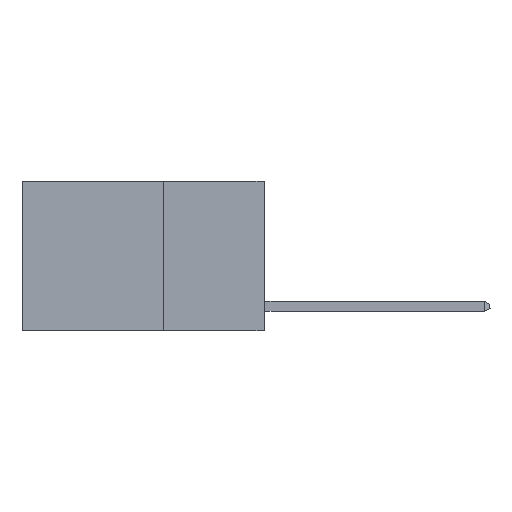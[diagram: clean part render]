
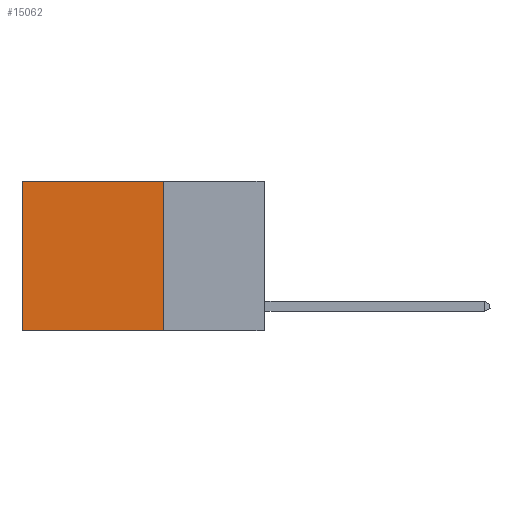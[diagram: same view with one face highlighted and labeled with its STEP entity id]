
A CAD part, left-side view. The second image highlights one B-rep face of the part: STEP entity #15062.
In plain terms, the highlighted planar face has unit normal (-1, 0, 0).
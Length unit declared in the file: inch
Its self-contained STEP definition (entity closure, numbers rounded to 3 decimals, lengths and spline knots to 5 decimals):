
#704 = CARTESIAN_POINT ( 'NONE',  ( 0.2625, 0.25, 0. ) ) ;
#871 = VECTOR ( 'NONE', #14915, 39.37008 ) ;
#1615 = ORIENTED_EDGE ( 'NONE', *, *, #5030, .F. ) ;
#2036 = CARTESIAN_POINT ( 'NONE',  ( 0.2625, 0.6, 0. ) ) ;
#3645 = VERTEX_POINT ( 'NONE', #19910 ) ;
#3768 = CARTESIAN_POINT ( 'NONE',  ( 0.2625, 0.25, 0. ) ) ;
#3844 = FACE_OUTER_BOUND ( 'NONE', #17387, .T. ) ;
#3846 = EDGE_CURVE ( 'NONE', #17988, #3645, #8798, .T. ) ;
#3856 = VERTEX_POINT ( 'NONE', #16458 ) ;
#4804 = LINE ( 'NONE', #2036, #16045 ) ;
#4992 = ORIENTED_EDGE ( 'NONE', *, *, #3846, .F. ) ;
#5030 = EDGE_CURVE ( 'NONE', #3645, #3856, #11576, .T. ) ;
#5071 = DIRECTION ( 'NONE',  ( 1., 0., 0. ) ) ;
#5619 = CARTESIAN_POINT ( 'NONE',  ( 0.2625, 0.25, 0. ) ) ;
#5846 = VECTOR ( 'NONE', #10046, 39.37008 ) ;
#6249 = CARTESIAN_POINT ( 'NONE',  ( 0.2625, 0.6, 0. ) ) ;
#6256 = VECTOR ( 'NONE', #14660, 39.37008 ) ;
#6425 = VERTEX_POINT ( 'NONE', #6249 ) ;
#8798 = LINE ( 'NONE', #5619, #5846 ) ;
#9884 = CARTESIAN_POINT ( 'NONE',  ( 0.2625, 0.25, 0. ) ) ;
#10046 = DIRECTION ( 'NONE',  ( 0., 0., -1. ) ) ;
#10089 = DIRECTION ( 'NONE',  ( 0., 0., -1. ) ) ;
#11225 = EDGE_CURVE ( 'NONE', #6425, #3856, #4804, .T. ) ;
#11576 = LINE ( 'NONE', #13328, #6256 ) ;
#12592 = AXIS2_PLACEMENT_3D ( 'NONE', #9884, #5071, #10089 ) ;
#13067 = ORIENTED_EDGE ( 'NONE', *, *, #16032, .T. ) ;
#13328 = CARTESIAN_POINT ( 'NONE',  ( 0.2625, 0.25, -0.37 ) ) ;
#14660 = DIRECTION ( 'NONE',  ( 0., 1., 0. ) ) ;
#14713 = LINE ( 'NONE', #704, #871 ) ;
#14885 = PLANE ( 'NONE',  #12592 ) ;
#14915 = DIRECTION ( 'NONE',  ( 0., 1., 0. ) ) ;
#15062 = ADVANCED_FACE ( 'NONE', ( #3844 ), #14885, .F. ) ;
#16032 = EDGE_CURVE ( 'NONE', #17988, #6425, #14713, .T. ) ;
#16045 = VECTOR ( 'NONE', #17282, 39.37008 ) ;
#16458 = CARTESIAN_POINT ( 'NONE',  ( 0.2625, 0.6, -0.37 ) ) ;
#16622 = ORIENTED_EDGE ( 'NONE', *, *, #11225, .T. ) ;
#17282 = DIRECTION ( 'NONE',  ( 0., 0., -1. ) ) ;
#17387 = EDGE_LOOP ( 'NONE', ( #16622, #1615, #4992, #13067 ) ) ;
#17988 = VERTEX_POINT ( 'NONE', #3768 ) ;
#19910 = CARTESIAN_POINT ( 'NONE',  ( 0.2625, 0.25, -0.37 ) ) ;
